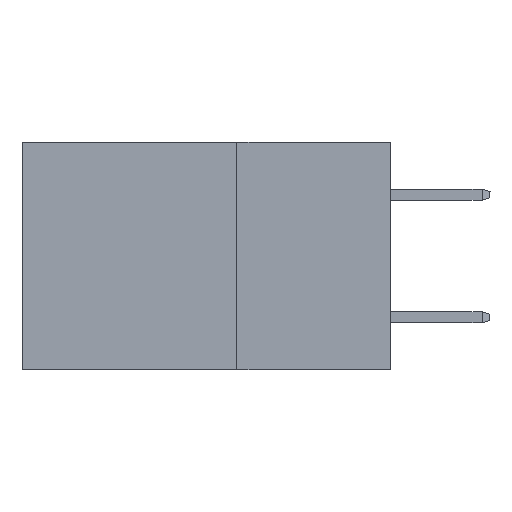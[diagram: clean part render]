
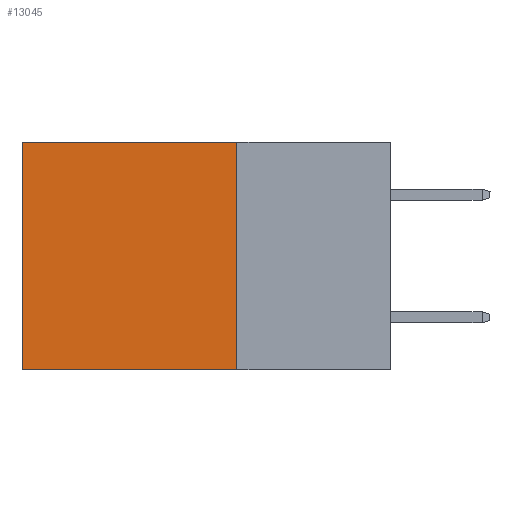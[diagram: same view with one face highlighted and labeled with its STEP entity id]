
A CAD part, left-side view. The second image highlights one B-rep face of the part: STEP entity #13045.
In plain terms, the highlighted planar face has unit normal (-1, 0, 0).
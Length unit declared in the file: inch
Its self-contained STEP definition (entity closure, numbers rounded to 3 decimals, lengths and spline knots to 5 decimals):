
#759 = VERTEX_POINT ( 'NONE', #11976 ) ;
#883 = VECTOR ( 'NONE', #17365, 39.37008 ) ;
#1946 = DIRECTION ( 'NONE',  ( 0., 0., -1. ) ) ;
#2438 = DIRECTION ( 'NONE',  ( 0., 0., -1. ) ) ;
#2583 = LINE ( 'NONE', #14780, #16063 ) ;
#4044 = ORIENTED_EDGE ( 'NONE', *, *, #6857, .F. ) ;
#4449 = VERTEX_POINT ( 'NONE', #9999 ) ;
#5447 = PLANE ( 'NONE',  #8771 ) ;
#5599 = LINE ( 'NONE', #8710, #883 ) ;
#6170 = EDGE_CURVE ( 'NONE', #4449, #759, #2583, .T. ) ;
#6596 = DIRECTION ( 'NONE',  ( 0., 0., -1. ) ) ;
#6857 = EDGE_CURVE ( 'NONE', #759, #21520, #11707, .T. ) ;
#7121 = EDGE_CURVE ( 'NONE', #4449, #12933, #5599, .T. ) ;
#7551 = VECTOR ( 'NONE', #6596, 39.37008 ) ;
#7658 = EDGE_CURVE ( 'NONE', #12933, #21520, #8641, .T. ) ;
#8220 = FACE_OUTER_BOUND ( 'NONE', #19610, .T. ) ;
#8641 = LINE ( 'NONE', #15315, #7551 ) ;
#8710 = CARTESIAN_POINT ( 'NONE',  ( 0.2875, 0.25, 0. ) ) ;
#8771 = AXIS2_PLACEMENT_3D ( 'NONE', #9010, #12523, #1946 ) ;
#9010 = CARTESIAN_POINT ( 'NONE',  ( 0.2875, 0.25, 0. ) ) ;
#9089 = ORIENTED_EDGE ( 'NONE', *, *, #7121, .T. ) ;
#9786 = DIRECTION ( 'NONE',  ( 0., 1., 0. ) ) ;
#9819 = ORIENTED_EDGE ( 'NONE', *, *, #6170, .F. ) ;
#9999 = CARTESIAN_POINT ( 'NONE',  ( 0.2875, 0.25, 0. ) ) ;
#11707 = LINE ( 'NONE', #21803, #19764 ) ;
#11726 = ORIENTED_EDGE ( 'NONE', *, *, #7658, .T. ) ;
#11976 = CARTESIAN_POINT ( 'NONE',  ( 0.2875, 0.25, -0.37 ) ) ;
#12523 = DIRECTION ( 'NONE',  ( 1., 0., 0. ) ) ;
#12933 = VERTEX_POINT ( 'NONE', #17307 ) ;
#13045 = ADVANCED_FACE ( 'NONE', ( #8220 ), #5447, .F. ) ;
#14780 = CARTESIAN_POINT ( 'NONE',  ( 0.2875, 0.25, 0. ) ) ;
#15315 = CARTESIAN_POINT ( 'NONE',  ( 0.2875, 0.6, 0. ) ) ;
#16063 = VECTOR ( 'NONE', #2438, 39.37008 ) ;
#17307 = CARTESIAN_POINT ( 'NONE',  ( 0.2875, 0.6, 0. ) ) ;
#17365 = DIRECTION ( 'NONE',  ( 0., 1., 0. ) ) ;
#19112 = CARTESIAN_POINT ( 'NONE',  ( 0.2875, 0.6, -0.37 ) ) ;
#19610 = EDGE_LOOP ( 'NONE', ( #11726, #4044, #9819, #9089 ) ) ;
#19764 = VECTOR ( 'NONE', #9786, 39.37008 ) ;
#21520 = VERTEX_POINT ( 'NONE', #19112 ) ;
#21803 = CARTESIAN_POINT ( 'NONE',  ( 0.2875, 0.25, -0.37 ) ) ;
